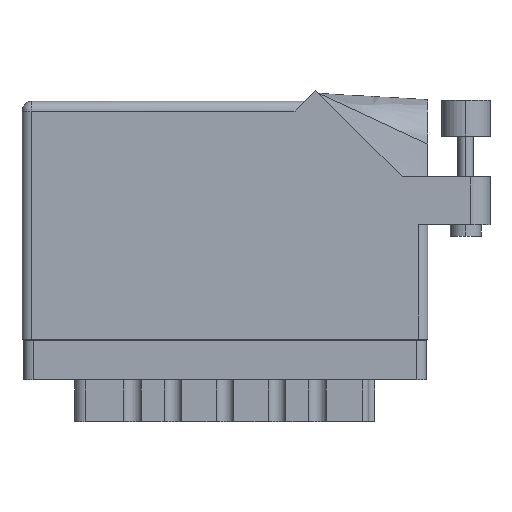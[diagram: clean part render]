
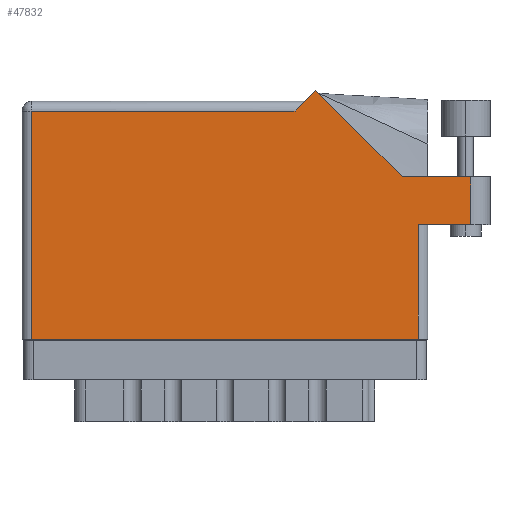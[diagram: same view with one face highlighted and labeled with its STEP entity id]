
A CAD part, front view. The second image highlights one B-rep face of the part: STEP entity #47832.
In plain terms, the highlighted face is planar.
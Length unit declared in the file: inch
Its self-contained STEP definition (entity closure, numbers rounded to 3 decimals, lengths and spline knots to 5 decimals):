
#996 = EDGE_CURVE ( 'NONE', #3185, #45168, #26214, .T. ) ;
#1270 = ORIENTED_EDGE ( 'NONE', *, *, #46331, .T. ) ;
#2055 = VERTEX_POINT ( 'NONE', #37068 ) ;
#3185 = VERTEX_POINT ( 'NONE', #47164 ) ;
#4364 = LINE ( 'NONE', #13333, #39927 ) ;
#4756 = EDGE_CURVE ( 'NONE', #44665, #21567, #33164, .T. ) ;
#5313 = ORIENTED_EDGE ( 'NONE', *, *, #40851, .T. ) ;
#5956 = VECTOR ( 'NONE', #44209, 39.37008 ) ;
#6065 = VECTOR ( 'NONE', #39798, 39.37008 ) ;
#7102 = LINE ( 'NONE', #28466, #5956 ) ;
#8033 = ORIENTED_EDGE ( 'NONE', *, *, #18653, .T. ) ;
#9948 = VERTEX_POINT ( 'NONE', #19116 ) ;
#10300 = LINE ( 'NONE', #41664, #37001 ) ;
#10400 = CARTESIAN_POINT ( 'NONE',  ( 0., 1.468, 0. ) ) ;
#11542 = VECTOR ( 'NONE', #37119, 39.37008 ) ;
#11709 = LINE ( 'NONE', #27208, #26019 ) ;
#12059 = ORIENTED_EDGE ( 'NONE', *, *, #30498, .T. ) ;
#12922 = VECTOR ( 'NONE', #21429, 39.37008 ) ;
#13148 = VERTEX_POINT ( 'NONE', #14074 ) ;
#13333 = CARTESIAN_POINT ( 'NONE',  ( 3.012, 1.044, 0. ) ) ;
#13769 = CARTESIAN_POINT ( 'NONE',  ( 2.55, 0.737, 0. ) ) ;
#14074 = CARTESIAN_POINT ( 'NONE',  ( 2.887, 1.044, 0. ) ) ;
#16293 = LINE ( 'NONE', #18027, #11542 ) ;
#16754 = DIRECTION ( 'NONE',  ( -1., 0., 0. ) ) ;
#17364 = CARTESIAN_POINT ( 'NONE',  ( 2.612, 0.737, 0. ) ) ;
#17754 = DIRECTION ( 'NONE',  ( 0., 1., 0. ) ) ;
#18027 = CARTESIAN_POINT ( 'NONE',  ( 0., 0., 0. ) ) ;
#18653 = EDGE_CURVE ( 'NONE', #9948, #44665, #48416, .T. ) ;
#19116 = CARTESIAN_POINT ( 'NONE',  ( 1.757, 1.468, 0. ) ) ;
#19177 = VERTEX_POINT ( 'NONE', #48492 ) ;
#19856 = ORIENTED_EDGE ( 'NONE', *, *, #4756, .T. ) ;
#21429 = DIRECTION ( 'NONE',  ( 0., -1., 0. ) ) ;
#21567 = VERTEX_POINT ( 'NONE', #34747 ) ;
#21584 = AXIS2_PLACEMENT_3D ( 'NONE', #35212, #46642, #16754 ) ;
#23085 = ORIENTED_EDGE ( 'NONE', *, *, #34156, .T. ) ;
#23176 = LINE ( 'NONE', #13769, #38056 ) ;
#25365 = ORIENTED_EDGE ( 'NONE', *, *, #996, .T. ) ;
#26019 = VECTOR ( 'NONE', #31718, 39.37008 ) ;
#26214 = LINE ( 'NONE', #17364, #6065 ) ;
#27208 = CARTESIAN_POINT ( 'NONE',  ( 1.819, 1.53, 0. ) ) ;
#28416 = PLANE ( 'NONE',  #21584 ) ;
#28466 = CARTESIAN_POINT ( 'NONE',  ( 2.44642, 1.044, 0. ) ) ;
#30128 = DIRECTION ( 'NONE',  ( -1., 0., 0. ) ) ;
#30498 = EDGE_CURVE ( 'NONE', #21567, #19177, #16293, .T. ) ;
#31718 = DIRECTION ( 'NONE',  ( -0.707, -0.707, 0. ) ) ;
#31932 = CARTESIAN_POINT ( 'NONE',  ( 2.44642, 1.044, 0. ) ) ;
#32510 = FACE_OUTER_BOUND ( 'NONE', #45869, .T. ) ;
#33164 = LINE ( 'NONE', #35389, #12922 ) ;
#33561 = VERTEX_POINT ( 'NONE', #31932 ) ;
#33748 = CARTESIAN_POINT ( 'NONE',  ( 2.887, 0.737, 0. ) ) ;
#33998 = EDGE_CURVE ( 'NONE', #45168, #13148, #10300, .T. ) ;
#34156 = EDGE_CURVE ( 'NONE', #2055, #9948, #11709, .T. ) ;
#34353 = DIRECTION ( 'NONE',  ( 0., 1., 0. ) ) ;
#34747 = CARTESIAN_POINT ( 'NONE',  ( 0.062, 0., 0. ) ) ;
#35212 = CARTESIAN_POINT ( 'NONE',  ( 0., 1.53, 0. ) ) ;
#35389 = CARTESIAN_POINT ( 'NONE',  ( 0.062, 0., 0. ) ) ;
#37001 = VECTOR ( 'NONE', #34353, 39.37008 ) ;
#37068 = CARTESIAN_POINT ( 'NONE',  ( 1.88971, 1.60071, 0. ) ) ;
#37119 = DIRECTION ( 'NONE',  ( 1., 0., 0. ) ) ;
#38056 = VECTOR ( 'NONE', #17754, 39.37008 ) ;
#38334 = VECTOR ( 'NONE', #30128, 39.37008 ) ;
#38925 = CARTESIAN_POINT ( 'NONE',  ( 0.062, 1.468, 0. ) ) ;
#39798 = DIRECTION ( 'NONE',  ( 1., 0., 0. ) ) ;
#39823 = ORIENTED_EDGE ( 'NONE', *, *, #41470, .T. ) ;
#39924 = DIRECTION ( 'NONE',  ( -1., 0., 0. ) ) ;
#39927 = VECTOR ( 'NONE', #39924, 39.37008 ) ;
#40851 = EDGE_CURVE ( 'NONE', #13148, #33561, #4364, .T. ) ;
#41470 = EDGE_CURVE ( 'NONE', #19177, #3185, #23176, .T. ) ;
#41664 = CARTESIAN_POINT ( 'NONE',  ( 2.887, 1.044, 0. ) ) ;
#44209 = DIRECTION ( 'NONE',  ( -0.707, 0.707, 0. ) ) ;
#44665 = VERTEX_POINT ( 'NONE', #38925 ) ;
#45168 = VERTEX_POINT ( 'NONE', #33748 ) ;
#45869 = EDGE_LOOP ( 'NONE', ( #25365, #48533, #5313, #1270, #23085, #8033, #19856, #12059, #39823 ) ) ;
#46331 = EDGE_CURVE ( 'NONE', #33561, #2055, #7102, .T. ) ;
#46642 = DIRECTION ( 'NONE',  ( 0., 0., -1. ) ) ;
#47164 = CARTESIAN_POINT ( 'NONE',  ( 2.55, 0.737, 0. ) ) ;
#47832 = ADVANCED_FACE ( 'NONE', ( #32510 ), #28416, .F. ) ;
#48416 = LINE ( 'NONE', #10400, #38334 ) ;
#48492 = CARTESIAN_POINT ( 'NONE',  ( 2.55, 0., 0. ) ) ;
#48533 = ORIENTED_EDGE ( 'NONE', *, *, #33998, .T. ) ;
